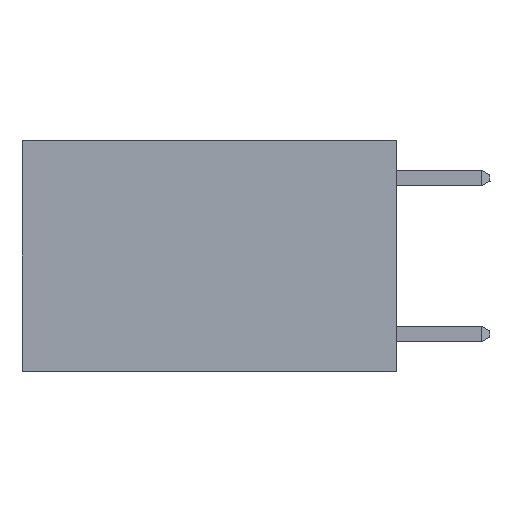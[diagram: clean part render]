
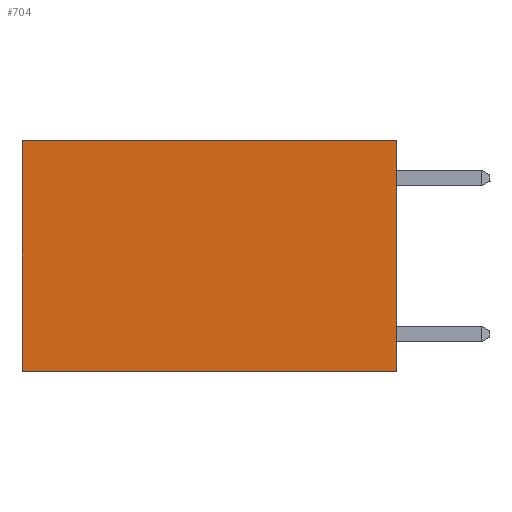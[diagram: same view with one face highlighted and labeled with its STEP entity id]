
A CAD part, left-side view. The second image highlights one B-rep face of the part: STEP entity #704.
In plain terms, the highlighted planar face has unit normal (-1, 0, 0).
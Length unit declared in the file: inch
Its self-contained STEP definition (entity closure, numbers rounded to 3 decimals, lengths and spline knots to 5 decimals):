
#122 = VERTEX_POINT ( 'NONE', #2734 ) ;
#184 = CARTESIAN_POINT ( 'NONE',  ( 0.2625, 0., -0.37 ) ) ;
#433 = LINE ( 'NONE', #1556, #4199 ) ;
#704 = ADVANCED_FACE ( 'NONE', ( #6605 ), #6215, .F. ) ;
#1266 = DIRECTION ( 'NONE',  ( 0., 0., -1. ) ) ;
#1338 = VERTEX_POINT ( 'NONE', #4409 ) ;
#1556 = CARTESIAN_POINT ( 'NONE',  ( 0.2625, 0., 0. ) ) ;
#1648 = LINE ( 'NONE', #8759, #5527 ) ;
#2287 = EDGE_CURVE ( 'NONE', #5905, #1338, #1648, .T. ) ;
#2635 = EDGE_LOOP ( 'NONE', ( #2917, #2835, #4684, #5201 ) ) ;
#2734 = CARTESIAN_POINT ( 'NONE',  ( 0.2625, 0., -0.37 ) ) ;
#2835 = ORIENTED_EDGE ( 'NONE', *, *, #9811, .F. ) ;
#2873 = DIRECTION ( 'NONE',  ( 1., 0., 0. ) ) ;
#2917 = ORIENTED_EDGE ( 'NONE', *, *, #8714, .T. ) ;
#2965 = VECTOR ( 'NONE', #7939, 39.37008 ) ;
#4093 = AXIS2_PLACEMENT_3D ( 'NONE', #10602, #2873, #1266 ) ;
#4199 = VECTOR ( 'NONE', #5124, 39.37008 ) ;
#4409 = CARTESIAN_POINT ( 'NONE',  ( 0.2625, 0.6, 0. ) ) ;
#4684 = ORIENTED_EDGE ( 'NONE', *, *, #7504, .F. ) ;
#5124 = DIRECTION ( 'NONE',  ( 0., 0., -1. ) ) ;
#5201 = ORIENTED_EDGE ( 'NONE', *, *, #2287, .T. ) ;
#5271 = LINE ( 'NONE', #8675, #2965 ) ;
#5527 = VECTOR ( 'NONE', #6231, 39.37008 ) ;
#5905 = VERTEX_POINT ( 'NONE', #9375 ) ;
#6215 = PLANE ( 'NONE',  #4093 ) ;
#6231 = DIRECTION ( 'NONE',  ( 0., 1., 0. ) ) ;
#6315 = VECTOR ( 'NONE', #6831, 39.37008 ) ;
#6605 = FACE_OUTER_BOUND ( 'NONE', #2635, .T. ) ;
#6831 = DIRECTION ( 'NONE',  ( 0., 1., 0. ) ) ;
#7504 = EDGE_CURVE ( 'NONE', #5905, #122, #433, .T. ) ;
#7939 = DIRECTION ( 'NONE',  ( 0., 0., -1. ) ) ;
#8675 = CARTESIAN_POINT ( 'NONE',  ( 0.2625, 0.6, 0. ) ) ;
#8714 = EDGE_CURVE ( 'NONE', #1338, #9499, #5271, .T. ) ;
#8759 = CARTESIAN_POINT ( 'NONE',  ( 0.2625, 0., 0. ) ) ;
#9108 = LINE ( 'NONE', #184, #6315 ) ;
#9375 = CARTESIAN_POINT ( 'NONE',  ( 0.2625, 0., 0. ) ) ;
#9499 = VERTEX_POINT ( 'NONE', #10565 ) ;
#9811 = EDGE_CURVE ( 'NONE', #122, #9499, #9108, .T. ) ;
#10565 = CARTESIAN_POINT ( 'NONE',  ( 0.2625, 0.6, -0.37 ) ) ;
#10602 = CARTESIAN_POINT ( 'NONE',  ( 0.2625, 0., 0. ) ) ;
